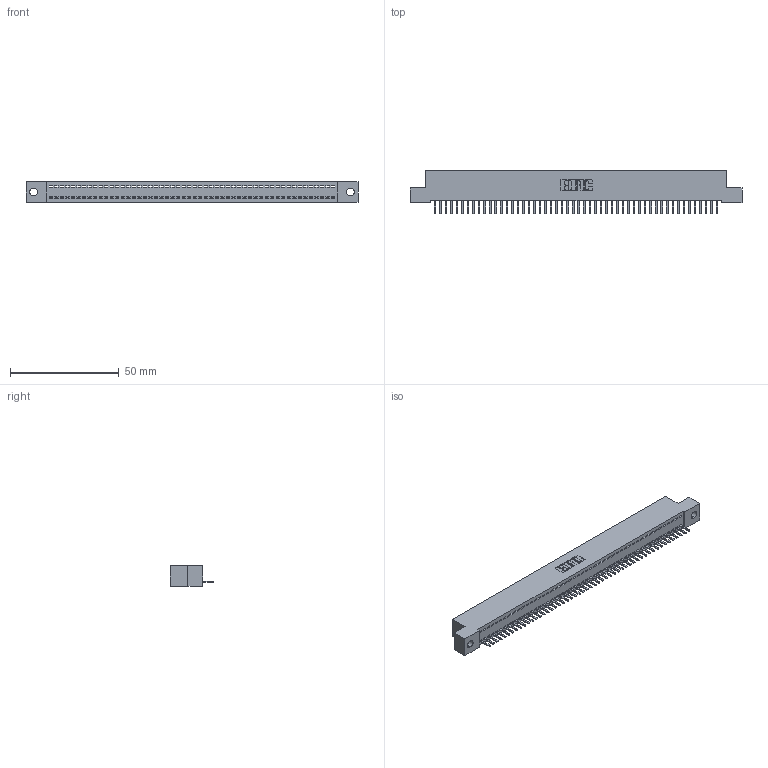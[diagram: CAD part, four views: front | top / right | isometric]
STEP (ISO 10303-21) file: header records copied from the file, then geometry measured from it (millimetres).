
FILE_DESCRIPTION (( 'STEP AP203' ), '1' );
FILE_NAME ('342-052-520-102.STEP', '2018-08-12T21:24:08', ( '' ), ( '' ), 'SwSTEP 2.0', 'SolidWorks 2016', '' );
FILE_SCHEMA (( 'CONFIG_CONTROL_DESIGN' ));
Length unit declared in the file: inch
Products named in the file (3): 342 Part_.128 Slot; 345-292-001_345-293-120; 342-052-520-102
Assembly tree (53 placements, depth 2):
  342-052-520-102
    342 Part_.128 Slot
    345-292-001_345-293-120  x52
Bounding box: 152.4 x 20.02 x 9.4 mm (x, y, z)
Volume: 13197.5 mm3; surface area: 18847.9 mm2
Topology: 53 solids, 53 shells, 3338 faces, 9879 edges, 6446 vertices
Faces by surface type: plane 2358, cylinder 980
Entity records: 30613 total; most frequent: CARTESIAN_POINT 5298, ORIENTED_EDGE 5274, DIRECTION 4437, EDGE_CURVE 2637, VECTOR 2505, LINE 2505, VERTEX_POINT 1754, AXIS2_PLACEMENT_3D 966
